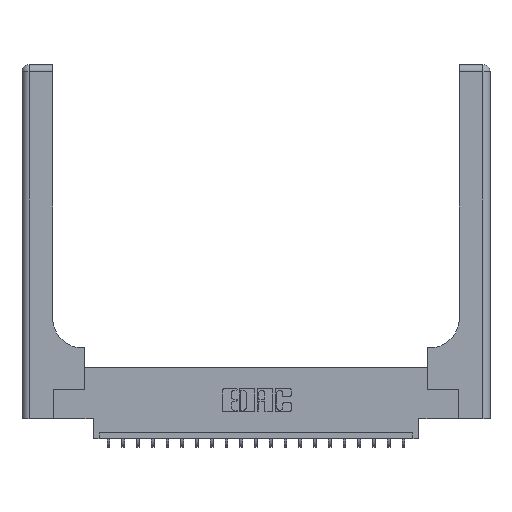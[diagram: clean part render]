
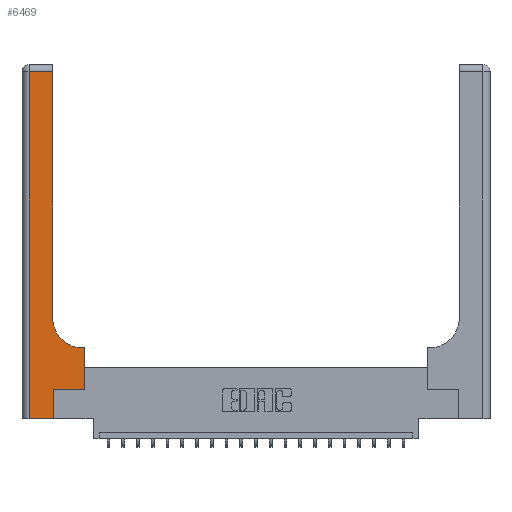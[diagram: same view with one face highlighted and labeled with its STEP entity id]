
A CAD part, top view. The second image highlights one B-rep face of the part: STEP entity #6469.
In plain terms, the highlighted planar face has unit normal (0, 0, 1).
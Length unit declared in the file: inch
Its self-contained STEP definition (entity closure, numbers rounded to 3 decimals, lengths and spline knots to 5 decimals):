
#67 = VERTEX_POINT ( 'NONE', #21491 ) ;
#94 = VECTOR ( 'NONE', #17258, 39.37008 ) ;
#193 = DIRECTION ( 'NONE',  ( 1., 0., 0. ) ) ;
#235 = VERTEX_POINT ( 'NONE', #10505 ) ;
#911 = VECTOR ( 'NONE', #2187, 39.37008 ) ;
#1091 = ORIENTED_EDGE ( 'NONE', *, *, #19557, .T. ) ;
#1314 = VERTEX_POINT ( 'NONE', #6782 ) ;
#1322 = CARTESIAN_POINT ( 'NONE',  ( 0.26, 0.85, 0.37 ) ) ;
#1451 = VERTEX_POINT ( 'NONE', #20493 ) ;
#2187 = DIRECTION ( 'NONE',  ( 0., 1., 0. ) ) ;
#2189 = LINE ( 'NONE', #2611, #11348 ) ;
#2611 = CARTESIAN_POINT ( 'NONE',  ( 0.06, 3., 0.37 ) ) ;
#2807 = CARTESIAN_POINT ( 'NONE',  ( 0.51, 0.6, 0.37 ) ) ;
#2946 = ORIENTED_EDGE ( 'NONE', *, *, #16800, .T. ) ;
#3353 = DIRECTION ( 'NONE',  ( 0., 1., 0. ) ) ;
#3915 = LINE ( 'NONE', #14183, #6014 ) ;
#4547 = VECTOR ( 'NONE', #15095, 39.37008 ) ;
#4748 = VECTOR ( 'NONE', #20700, 39.37008 ) ;
#5788 = LINE ( 'NONE', #18940, #911 ) ;
#5889 = CARTESIAN_POINT ( 'NONE',  ( 0.265, 0.25, 0.37 ) ) ;
#5950 = LINE ( 'NONE', #12715, #10966 ) ;
#6014 = VECTOR ( 'NONE', #21008, 39.37008 ) ;
#6347 = CARTESIAN_POINT ( 'NONE',  ( 0.51, 0.85, 0.37 ) ) ;
#6467 = VERTEX_POINT ( 'NONE', #14819 ) ;
#6469 = ADVANCED_FACE ( 'NONE', ( #18224 ), #9790, .F. ) ;
#6782 = CARTESIAN_POINT ( 'NONE',  ( 0.265, 0., 0.37 ) ) ;
#6853 = CARTESIAN_POINT ( 'NONE',  ( 0.265, 0.25, 0.37 ) ) ;
#7321 = LINE ( 'NONE', #5889, #4748 ) ;
#7524 = EDGE_CURVE ( 'NONE', #67, #1451, #5788, .T. ) ;
#7530 = AXIS2_PLACEMENT_3D ( 'NONE', #6347, #16646, #193 ) ;
#8724 = CARTESIAN_POINT ( 'NONE',  ( 0.26, 0.6, 0.37 ) ) ;
#8865 = DIRECTION ( 'NONE',  ( 0., -1., 0. ) ) ;
#8917 = EDGE_LOOP ( 'NONE', ( #2946, #1091, #16266, #9962, #10736, #18417, #11407, #21092, #10126 ) ) ;
#9338 = VERTEX_POINT ( 'NONE', #1322 ) ;
#9790 = PLANE ( 'NONE',  #14339 ) ;
#9892 = VECTOR ( 'NONE', #3353, 39.37008 ) ;
#9943 = CARTESIAN_POINT ( 'NONE',  ( 0., 0., 0.37 ) ) ;
#9962 = ORIENTED_EDGE ( 'NONE', *, *, #12867, .T. ) ;
#10126 = ORIENTED_EDGE ( 'NONE', *, *, #19054, .T. ) ;
#10505 = CARTESIAN_POINT ( 'NONE',  ( 0.06, 0., 0.37 ) ) ;
#10736 = ORIENTED_EDGE ( 'NONE', *, *, #14701, .T. ) ;
#10966 = VECTOR ( 'NONE', #11182, 39.37008 ) ;
#11182 = DIRECTION ( 'NONE',  ( -1., 0., 0. ) ) ;
#11340 = VERTEX_POINT ( 'NONE', #13670 ) ;
#11348 = VECTOR ( 'NONE', #8865, 39.37008 ) ;
#11407 = ORIENTED_EDGE ( 'NONE', *, *, #7524, .T. ) ;
#12715 = CARTESIAN_POINT ( 'NONE',  ( 0., 2.94, 0.37 ) ) ;
#12867 = EDGE_CURVE ( 'NONE', #235, #1314, #15201, .T. ) ;
#13281 = DIRECTION ( 'NONE',  ( 0., 0., -1. ) ) ;
#13634 = LINE ( 'NONE', #8724, #94 ) ;
#13670 = CARTESIAN_POINT ( 'NONE',  ( 0.06, 2.94, 0.37 ) ) ;
#13763 = CIRCLE ( 'NONE', #7530, 0.25 ) ;
#14183 = CARTESIAN_POINT ( 'NONE',  ( 0.265, 0., 0.37 ) ) ;
#14339 = AXIS2_PLACEMENT_3D ( 'NONE', #19994, #13281, #21530 ) ;
#14701 = EDGE_CURVE ( 'NONE', #1314, #21416, #3915, .T. ) ;
#14819 = CARTESIAN_POINT ( 'NONE',  ( 0.26, 2.94, 0.37 ) ) ;
#14837 = VERTEX_POINT ( 'NONE', #2807 ) ;
#15095 = DIRECTION ( 'NONE',  ( 1., 0., 0. ) ) ;
#15201 = LINE ( 'NONE', #9943, #4547 ) ;
#16266 = ORIENTED_EDGE ( 'NONE', *, *, #19240, .T. ) ;
#16646 = DIRECTION ( 'NONE',  ( 0., 0., -1. ) ) ;
#16800 = EDGE_CURVE ( 'NONE', #9338, #6467, #20122, .T. ) ;
#16825 = EDGE_CURVE ( 'NONE', #1451, #14837, #13634, .T. ) ;
#17258 = DIRECTION ( 'NONE',  ( -1., 0., 0. ) ) ;
#18224 = FACE_OUTER_BOUND ( 'NONE', #8917, .T. ) ;
#18246 = CARTESIAN_POINT ( 'NONE',  ( 0.26, 3., 0.37 ) ) ;
#18417 = ORIENTED_EDGE ( 'NONE', *, *, #21203, .T. ) ;
#18940 = CARTESIAN_POINT ( 'NONE',  ( 0.528, 0.25, 0.37 ) ) ;
#19054 = EDGE_CURVE ( 'NONE', #14837, #9338, #13763, .T. ) ;
#19240 = EDGE_CURVE ( 'NONE', #11340, #235, #2189, .T. ) ;
#19557 = EDGE_CURVE ( 'NONE', #6467, #11340, #5950, .T. ) ;
#19994 = CARTESIAN_POINT ( 'NONE',  ( 0., 3., 0.37 ) ) ;
#20122 = LINE ( 'NONE', #18246, #9892 ) ;
#20493 = CARTESIAN_POINT ( 'NONE',  ( 0.528, 0.6, 0.37 ) ) ;
#20700 = DIRECTION ( 'NONE',  ( 1., 0., 0. ) ) ;
#21008 = DIRECTION ( 'NONE',  ( 0., 1., 0. ) ) ;
#21092 = ORIENTED_EDGE ( 'NONE', *, *, #16825, .T. ) ;
#21203 = EDGE_CURVE ( 'NONE', #21416, #67, #7321, .T. ) ;
#21416 = VERTEX_POINT ( 'NONE', #6853 ) ;
#21491 = CARTESIAN_POINT ( 'NONE',  ( 0.528, 0.25, 0.37 ) ) ;
#21530 = DIRECTION ( 'NONE',  ( -1., 0., 0. ) ) ;
